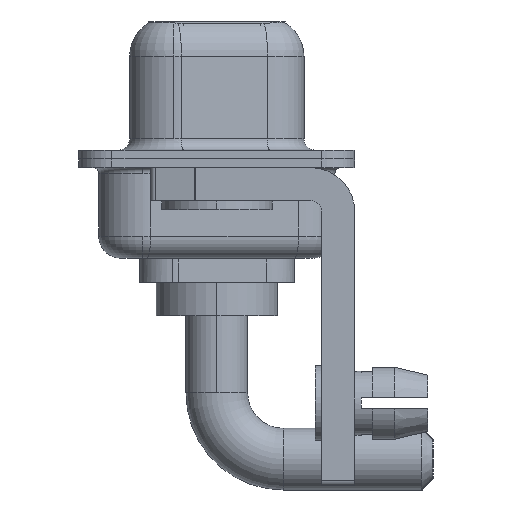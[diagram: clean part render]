
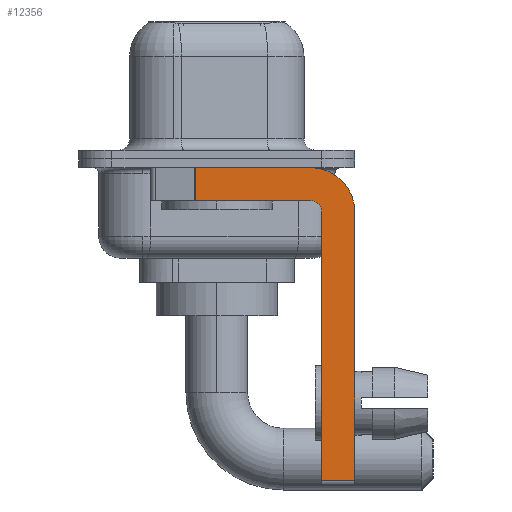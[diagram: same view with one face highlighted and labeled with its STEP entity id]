
A CAD part, left-side view. The second image highlights one B-rep face of the part: STEP entity #12356.
In plain terms, the highlighted planar face has unit normal (-1, 0, 0).
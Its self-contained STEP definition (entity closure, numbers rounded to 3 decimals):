
#684 = VERTEX_POINT ( 'NONE', #11415 ) ;
#721 = CARTESIAN_POINT ( 'NONE',  ( -2.9, -4.25, -1.9 ) ) ;
#955 = LINE ( 'NONE', #10921, #1670 ) ;
#1364 = DIRECTION ( 'NONE',  ( 0., -1., 0. ) ) ;
#1670 = VECTOR ( 'NONE', #4691, 1000. ) ;
#1697 = LINE ( 'NONE', #13804, #9429 ) ;
#2258 = EDGE_CURVE ( 'NONE', #7060, #12832, #1697, .T. ) ;
#2392 = VECTOR ( 'NONE', #7367, 1000. ) ;
#2421 = ORIENTED_EDGE ( 'NONE', *, *, #2600, .T. ) ;
#2564 = EDGE_CURVE ( 'NONE', #12207, #684, #13388, .T. ) ;
#2600 = EDGE_CURVE ( 'NONE', #7060, #2858, #3393, .T. ) ;
#2858 = VERTEX_POINT ( 'NONE', #5486 ) ;
#3142 = AXIS2_PLACEMENT_3D ( 'NONE', #10822, #9410, #14660 ) ;
#3393 = LINE ( 'NONE', #9837, #13634 ) ;
#3560 = VECTOR ( 'NONE', #12090, 1000. ) ;
#3933 = ORIENTED_EDGE ( 'NONE', *, *, #11759, .T. ) ;
#4034 = CARTESIAN_POINT ( 'NONE',  ( -2.9, -4.75, -14.55 ) ) ;
#4047 = EDGE_CURVE ( 'NONE', #11838, #4679, #955, .T. ) ;
#4400 = ORIENTED_EDGE ( 'NONE', *, *, #2258, .F. ) ;
#4668 = FACE_OUTER_BOUND ( 'NONE', #4943, .T. ) ;
#4679 = VERTEX_POINT ( 'NONE', #15138 ) ;
#4691 = DIRECTION ( 'NONE',  ( 0., 0., -1. ) ) ;
#4943 = EDGE_LOOP ( 'NONE', ( #4400, #2421, #15617, #9055, #6290, #3933, #15998, #12851 ) ) ;
#5206 = DIRECTION ( 'NONE',  ( 0., 0., -1. ) ) ;
#5486 = CARTESIAN_POINT ( 'NONE',  ( -2.9, 0.978, -1.9 ) ) ;
#6059 = DIRECTION ( 'NONE',  ( 0., 0., -1. ) ) ;
#6290 = ORIENTED_EDGE ( 'NONE', *, *, #2564, .F. ) ;
#6725 = EDGE_CURVE ( 'NONE', #9191, #2858, #10613, .T. ) ;
#6730 = CARTESIAN_POINT ( 'NONE',  ( -2.9, -6.25, -2.4 ) ) ;
#7060 = VERTEX_POINT ( 'NONE', #14183 ) ;
#7367 = DIRECTION ( 'NONE',  ( 0., 0., 1. ) ) ;
#7575 = DIRECTION ( 'NONE',  ( 1., 0., 0. ) ) ;
#9055 = ORIENTED_EDGE ( 'NONE', *, *, #14886, .F. ) ;
#9191 = VERTEX_POINT ( 'NONE', #15114 ) ;
#9410 = DIRECTION ( 'NONE',  ( 1., 0., 0. ) ) ;
#9429 = VECTOR ( 'NONE', #1364, 1000. ) ;
#9658 = PLANE ( 'NONE',  #3142 ) ;
#9837 = CARTESIAN_POINT ( 'NONE',  ( -2.9, 0.978, -1.9 ) ) ;
#9943 = CIRCLE ( 'NONE', #12841, 2. ) ;
#10204 = CIRCLE ( 'NONE', #13879, 0.5 ) ;
#10298 = CARTESIAN_POINT ( 'NONE',  ( -2.9, -4.25, -2.4 ) ) ;
#10613 = LINE ( 'NONE', #721, #3560 ) ;
#10822 = CARTESIAN_POINT ( 'NONE',  ( -2.9, -4.25, -2.4 ) ) ;
#10917 = CARTESIAN_POINT ( 'NONE',  ( -2.9, -4.75, -14.8 ) ) ;
#10921 = CARTESIAN_POINT ( 'NONE',  ( -2.9, -6.25, -2.4 ) ) ;
#10923 = VECTOR ( 'NONE', #11915, 1000. ) ;
#11046 = CARTESIAN_POINT ( 'NONE',  ( -2.9, -4.25, -2.4 ) ) ;
#11415 = CARTESIAN_POINT ( 'NONE',  ( -2.9, -4.75, -2.4 ) ) ;
#11759 = EDGE_CURVE ( 'NONE', #12207, #4679, #13065, .T. ) ;
#11835 = CARTESIAN_POINT ( 'NONE',  ( -2.9, -4.25, -14.55 ) ) ;
#11838 = VERTEX_POINT ( 'NONE', #6730 ) ;
#11915 = DIRECTION ( 'NONE',  ( 0., -1., 0. ) ) ;
#12090 = DIRECTION ( 'NONE',  ( 0., 1., 0. ) ) ;
#12207 = VERTEX_POINT ( 'NONE', #4034 ) ;
#12356 = ADVANCED_FACE ( 'NONE', ( #4668 ), #9658, .F. ) ;
#12453 = CARTESIAN_POINT ( 'NONE',  ( -2.9, -4.25, -0.4 ) ) ;
#12832 = VERTEX_POINT ( 'NONE', #12453 ) ;
#12841 = AXIS2_PLACEMENT_3D ( 'NONE', #10298, #7575, #5206 ) ;
#12851 = ORIENTED_EDGE ( 'NONE', *, *, #15029, .F. ) ;
#13065 = LINE ( 'NONE', #11835, #10923 ) ;
#13388 = LINE ( 'NONE', #10917, #2392 ) ;
#13634 = VECTOR ( 'NONE', #6059, 1000. ) ;
#13804 = CARTESIAN_POINT ( 'NONE',  ( -2.9, 3., -0.4 ) ) ;
#13879 = AXIS2_PLACEMENT_3D ( 'NONE', #11046, #16108, #16033 ) ;
#14183 = CARTESIAN_POINT ( 'NONE',  ( -2.9, 0.978, -0.4 ) ) ;
#14660 = DIRECTION ( 'NONE',  ( 0., 0., -1. ) ) ;
#14886 = EDGE_CURVE ( 'NONE', #684, #9191, #10204, .T. ) ;
#15029 = EDGE_CURVE ( 'NONE', #12832, #11838, #9943, .T. ) ;
#15114 = CARTESIAN_POINT ( 'NONE',  ( -2.9, -4.25, -1.9 ) ) ;
#15138 = CARTESIAN_POINT ( 'NONE',  ( -2.9, -6.25, -14.55 ) ) ;
#15617 = ORIENTED_EDGE ( 'NONE', *, *, #6725, .F. ) ;
#15998 = ORIENTED_EDGE ( 'NONE', *, *, #4047, .F. ) ;
#16033 = DIRECTION ( 'NONE',  ( 0., 0., 1. ) ) ;
#16108 = DIRECTION ( 'NONE',  ( -1., 0., 0. ) ) ;
